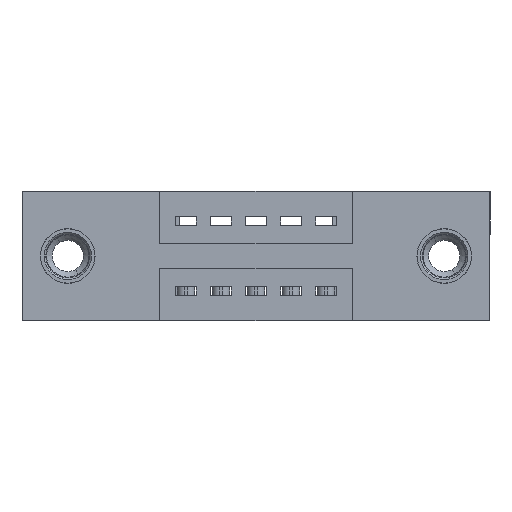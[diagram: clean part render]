
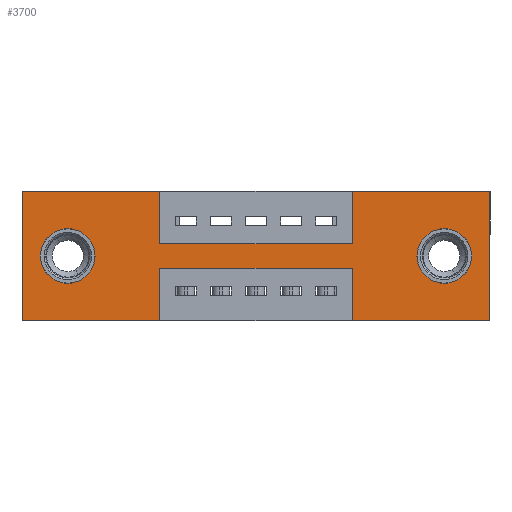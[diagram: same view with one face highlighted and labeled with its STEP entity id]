
A CAD part, front view. The second image highlights one B-rep face of the part: STEP entity #3700.
In plain terms, the highlighted planar face has unit normal (0, -1, 0).
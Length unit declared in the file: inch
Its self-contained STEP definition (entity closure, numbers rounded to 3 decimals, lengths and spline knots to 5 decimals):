
#4 = ORIENTED_EDGE ( 'NONE', *, *, #5868, .F. ) ;
#80 = CARTESIAN_POINT ( 'NONE',  ( 0., 0., -0.37 ) ) ;
#98 = ORIENTED_EDGE ( 'NONE', *, *, #11701, .T. ) ;
#125 = DIRECTION ( 'NONE',  ( 1., 0., 0. ) ) ;
#357 = VERTEX_POINT ( 'NONE', #1747 ) ;
#395 = DIRECTION ( 'NONE',  ( 1., 0., 0. ) ) ;
#529 = DIRECTION ( 'NONE',  ( 0., 1., 0. ) ) ;
#605 = VERTEX_POINT ( 'NONE', #7544 ) ;
#756 = CARTESIAN_POINT ( 'NONE',  ( 0.9425, 0., 0. ) ) ;
#835 = CARTESIAN_POINT ( 'NONE',  ( 0.13, 0., -0.263 ) ) ;
#1052 = VECTOR ( 'NONE', #13262, 39.37008 ) ;
#1199 = CARTESIAN_POINT ( 'NONE',  ( 0.9425, 0., -0.15 ) ) ;
#1301 = LINE ( 'NONE', #1532, #4538 ) ;
#1306 = DIRECTION ( 'NONE',  ( 0., 0., -1. ) ) ;
#1358 = DIRECTION ( 'NONE',  ( 0., 0., -1. ) ) ;
#1398 = ORIENTED_EDGE ( 'NONE', *, *, #7210, .T. ) ;
#1415 = ORIENTED_EDGE ( 'NONE', *, *, #4636, .T. ) ;
#1532 = CARTESIAN_POINT ( 'NONE',  ( 0.3925, 0., -0.22 ) ) ;
#1661 = LINE ( 'NONE', #9328, #8139 ) ;
#1747 = CARTESIAN_POINT ( 'NONE',  ( 0.3925, 0., -0.37 ) ) ;
#1788 = DIRECTION ( 'NONE',  ( 0., 0., 1. ) ) ;
#1969 = VECTOR ( 'NONE', #3555, 39.37008 ) ;
#2128 = PLANE ( 'NONE',  #3436 ) ;
#2135 = CIRCLE ( 'NONE', #3594, 0.078 ) ;
#2339 = EDGE_CURVE ( 'NONE', #5070, #11275, #11337, .T. ) ;
#2543 = EDGE_CURVE ( 'NONE', #3737, #10654, #7287, .T. ) ;
#2865 = ORIENTED_EDGE ( 'NONE', *, *, #4451, .F. ) ;
#3173 = CARTESIAN_POINT ( 'NONE',  ( 0., 0., -0.37 ) ) ;
#3312 = EDGE_CURVE ( 'NONE', #9991, #605, #1301, .T. ) ;
#3329 = EDGE_CURVE ( 'NONE', #3566, #5070, #6134, .T. ) ;
#3383 = DIRECTION ( 'NONE',  ( 0., 0., 1. ) ) ;
#3418 = EDGE_CURVE ( 'NONE', #605, #357, #7768, .T. ) ;
#3436 = AXIS2_PLACEMENT_3D ( 'NONE', #3173, #12492, #10403 ) ;
#3555 = DIRECTION ( 'NONE',  ( -1., 0., 0. ) ) ;
#3566 = VERTEX_POINT ( 'NONE', #756 ) ;
#3594 = AXIS2_PLACEMENT_3D ( 'NONE', #10072, #3841, #8085 ) ;
#3624 = DIRECTION ( 'NONE',  ( 0., 0., 1. ) ) ;
#3646 = ORIENTED_EDGE ( 'NONE', *, *, #8676, .F. ) ;
#3700 = ADVANCED_FACE ( 'NONE', ( #5000, #6607, #12465 ), #2128, .T. ) ;
#3737 = VERTEX_POINT ( 'NONE', #80 ) ;
#3820 = LINE ( 'NONE', #8761, #1052 ) ;
#3841 = DIRECTION ( 'NONE',  ( 0., 1., 0. ) ) ;
#4401 = CARTESIAN_POINT ( 'NONE',  ( 0., 0., 0. ) ) ;
#4451 = EDGE_CURVE ( 'NONE', #10654, #8837, #1661, .T. ) ;
#4538 = VECTOR ( 'NONE', #10668, 39.37008 ) ;
#4569 = AXIS2_PLACEMENT_3D ( 'NONE', #10503, #12652, #6417 ) ;
#4589 = EDGE_LOOP ( 'NONE', ( #10052, #10746, #10497, #8423, #12085, #13440, #6890, #4, #5794, #2865, #4849, #3646 ) ) ;
#4621 = DIRECTION ( 'NONE',  ( 0., 0., -1. ) ) ;
#4636 = EDGE_CURVE ( 'NONE', #12450, #6269, #5852, .T. ) ;
#4788 = CIRCLE ( 'NONE', #5487, 0.078 ) ;
#4849 = ORIENTED_EDGE ( 'NONE', *, *, #2543, .F. ) ;
#5000 = FACE_BOUND ( 'NONE', #9171, .T. ) ;
#5070 = VERTEX_POINT ( 'NONE', #9525 ) ;
#5487 = AXIS2_PLACEMENT_3D ( 'NONE', #11572, #10605, #11651 ) ;
#5625 = CARTESIAN_POINT ( 'NONE',  ( 0.3925, 0., -0.15 ) ) ;
#5794 = ORIENTED_EDGE ( 'NONE', *, *, #10147, .F. ) ;
#5852 = CIRCLE ( 'NONE', #12374, 0.078 ) ;
#5868 = EDGE_CURVE ( 'NONE', #11946, #7609, #8332, .T. ) ;
#5884 = VECTOR ( 'NONE', #12853, 39.37008 ) ;
#6134 = LINE ( 'NONE', #11719, #8565 ) ;
#6269 = VERTEX_POINT ( 'NONE', #10727 ) ;
#6417 = DIRECTION ( 'NONE',  ( 0., 0., -1. ) ) ;
#6607 = FACE_BOUND ( 'NONE', #10532, .T. ) ;
#6788 = VECTOR ( 'NONE', #1788, 39.37008 ) ;
#6842 = CARTESIAN_POINT ( 'NONE',  ( 0.9425, 0., 0. ) ) ;
#6890 = ORIENTED_EDGE ( 'NONE', *, *, #11348, .F. ) ;
#7210 = EDGE_CURVE ( 'NONE', #7254, #11490, #2135, .T. ) ;
#7254 = VERTEX_POINT ( 'NONE', #835 ) ;
#7287 = LINE ( 'NONE', #9811, #12143 ) ;
#7544 = CARTESIAN_POINT ( 'NONE',  ( 0.3925, 0., -0.22 ) ) ;
#7609 = VERTEX_POINT ( 'NONE', #1199 ) ;
#7768 = LINE ( 'NONE', #12906, #10359 ) ;
#7822 = LINE ( 'NONE', #10636, #13018 ) ;
#8085 = DIRECTION ( 'NONE',  ( 0., 0., 1. ) ) ;
#8139 = VECTOR ( 'NONE', #125, 39.37008 ) ;
#8227 = CARTESIAN_POINT ( 'NONE',  ( 0.3925, 0., -0.15 ) ) ;
#8332 = LINE ( 'NONE', #5625, #5884 ) ;
#8423 = ORIENTED_EDGE ( 'NONE', *, *, #11741, .F. ) ;
#8523 = ORIENTED_EDGE ( 'NONE', *, *, #8951, .T. ) ;
#8565 = VECTOR ( 'NONE', #395, 39.37008 ) ;
#8620 = CARTESIAN_POINT ( 'NONE',  ( 0.9425, 0., -0.37 ) ) ;
#8676 = EDGE_CURVE ( 'NONE', #357, #3737, #3820, .T. ) ;
#8761 = CARTESIAN_POINT ( 'NONE',  ( 0., 0., -0.37 ) ) ;
#8837 = VERTEX_POINT ( 'NONE', #9261 ) ;
#8911 = VECTOR ( 'NONE', #3383, 39.37008 ) ;
#8951 = EDGE_CURVE ( 'NONE', #11490, #7254, #4788, .T. ) ;
#9171 = EDGE_LOOP ( 'NONE', ( #98, #1415 ) ) ;
#9246 = CIRCLE ( 'NONE', #4569, 0.078 ) ;
#9261 = CARTESIAN_POINT ( 'NONE',  ( 0.3925, 0., 0. ) ) ;
#9328 = CARTESIAN_POINT ( 'NONE',  ( 0., 0., 0. ) ) ;
#9404 = LINE ( 'NONE', #6842, #6788 ) ;
#9419 = LINE ( 'NONE', #8620, #8911 ) ;
#9525 = CARTESIAN_POINT ( 'NONE',  ( 1.335, 0., 0. ) ) ;
#9697 = CARTESIAN_POINT ( 'NONE',  ( 0., 0., -0.37 ) ) ;
#9811 = CARTESIAN_POINT ( 'NONE',  ( 0., 0., 0. ) ) ;
#9813 = CARTESIAN_POINT ( 'NONE',  ( 1.205, 0., -0.185 ) ) ;
#9900 = LINE ( 'NONE', #9697, #1969 ) ;
#9991 = VERTEX_POINT ( 'NONE', #10690 ) ;
#10052 = ORIENTED_EDGE ( 'NONE', *, *, #3418, .F. ) ;
#10072 = CARTESIAN_POINT ( 'NONE',  ( 0.13, 0., -0.185 ) ) ;
#10147 = EDGE_CURVE ( 'NONE', #8837, #11946, #7822, .T. ) ;
#10359 = VECTOR ( 'NONE', #1358, 39.37008 ) ;
#10403 = DIRECTION ( 'NONE',  ( 0., 0., -1. ) ) ;
#10497 = ORIENTED_EDGE ( 'NONE', *, *, #11095, .F. ) ;
#10503 = CARTESIAN_POINT ( 'NONE',  ( 1.205, 0., -0.185 ) ) ;
#10532 = EDGE_LOOP ( 'NONE', ( #8523, #1398 ) ) ;
#10605 = DIRECTION ( 'NONE',  ( 0., 1., 0. ) ) ;
#10636 = CARTESIAN_POINT ( 'NONE',  ( 0.3925, 0., 0. ) ) ;
#10654 = VERTEX_POINT ( 'NONE', #4401 ) ;
#10668 = DIRECTION ( 'NONE',  ( -1., 0., 0. ) ) ;
#10690 = CARTESIAN_POINT ( 'NONE',  ( 0.9425, 0., -0.22 ) ) ;
#10727 = CARTESIAN_POINT ( 'NONE',  ( 1.205, 0., -0.107 ) ) ;
#10746 = ORIENTED_EDGE ( 'NONE', *, *, #3312, .F. ) ;
#11095 = EDGE_CURVE ( 'NONE', #13227, #9991, #9419, .T. ) ;
#11243 = CARTESIAN_POINT ( 'NONE',  ( 0.13, 0., -0.107 ) ) ;
#11275 = VERTEX_POINT ( 'NONE', #12932 ) ;
#11337 = LINE ( 'NONE', #12728, #11984 ) ;
#11348 = EDGE_CURVE ( 'NONE', #7609, #3566, #9404, .T. ) ;
#11490 = VERTEX_POINT ( 'NONE', #11243 ) ;
#11572 = CARTESIAN_POINT ( 'NONE',  ( 0.13, 0., -0.185 ) ) ;
#11651 = DIRECTION ( 'NONE',  ( 0., 0., 1. ) ) ;
#11701 = EDGE_CURVE ( 'NONE', #6269, #12450, #9246, .T. ) ;
#11719 = CARTESIAN_POINT ( 'NONE',  ( 0., 0., 0. ) ) ;
#11741 = EDGE_CURVE ( 'NONE', #11275, #13227, #9900, .T. ) ;
#11946 = VERTEX_POINT ( 'NONE', #8227 ) ;
#11984 = VECTOR ( 'NONE', #1306, 39.37008 ) ;
#12085 = ORIENTED_EDGE ( 'NONE', *, *, #2339, .F. ) ;
#12143 = VECTOR ( 'NONE', #3624, 39.37008 ) ;
#12196 = CARTESIAN_POINT ( 'NONE',  ( 0.9425, 0., -0.37 ) ) ;
#12374 = AXIS2_PLACEMENT_3D ( 'NONE', #9813, #529, #4621 ) ;
#12450 = VERTEX_POINT ( 'NONE', #12632 ) ;
#12465 = FACE_OUTER_BOUND ( 'NONE', #4589, .T. ) ;
#12492 = DIRECTION ( 'NONE',  ( 0., -1., 0. ) ) ;
#12632 = CARTESIAN_POINT ( 'NONE',  ( 1.205, 0., -0.263 ) ) ;
#12652 = DIRECTION ( 'NONE',  ( 0., 1., 0. ) ) ;
#12728 = CARTESIAN_POINT ( 'NONE',  ( 1.335, 0., 0. ) ) ;
#12853 = DIRECTION ( 'NONE',  ( 1., 0., 0. ) ) ;
#12906 = CARTESIAN_POINT ( 'NONE',  ( 0.3925, 0., -0.37 ) ) ;
#12932 = CARTESIAN_POINT ( 'NONE',  ( 1.335, 0., -0.37 ) ) ;
#12970 = DIRECTION ( 'NONE',  ( 0., 0., -1. ) ) ;
#13018 = VECTOR ( 'NONE', #12970, 39.37008 ) ;
#13227 = VERTEX_POINT ( 'NONE', #12196 ) ;
#13262 = DIRECTION ( 'NONE',  ( -1., 0., 0. ) ) ;
#13440 = ORIENTED_EDGE ( 'NONE', *, *, #3329, .F. ) ;
